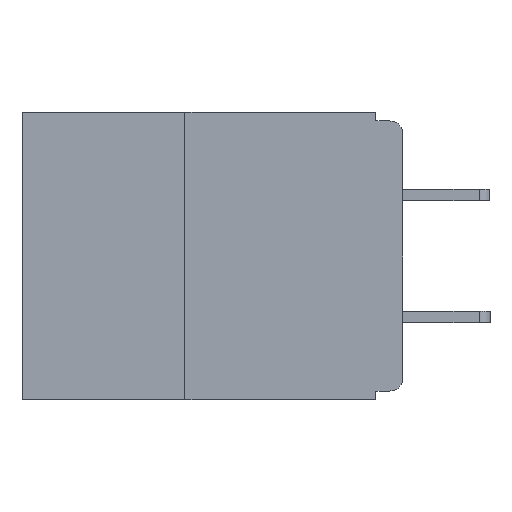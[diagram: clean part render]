
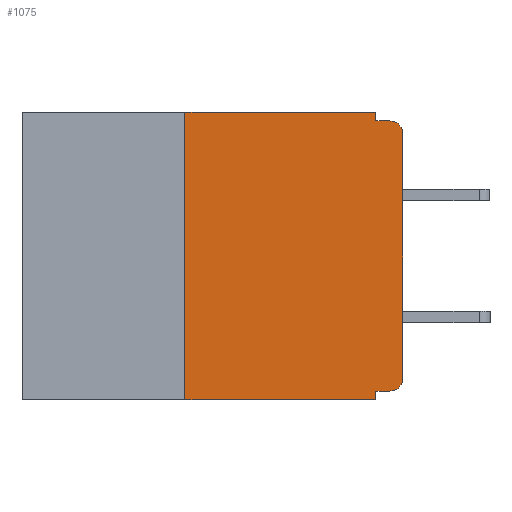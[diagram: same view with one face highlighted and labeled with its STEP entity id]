
A CAD part, left-side view. The second image highlights one B-rep face of the part: STEP entity #1075.
In plain terms, the highlighted planar face has unit normal (-1, 0, 0).
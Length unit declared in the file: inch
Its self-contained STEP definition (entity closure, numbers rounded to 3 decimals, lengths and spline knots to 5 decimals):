
#1011 = EDGE_CURVE ( 'NONE', #8571, #1750, #12185, .T. ) ;
#1016 = AXIS2_PLACEMENT_3D ( 'NONE', #9507, #27413, #12088 ) ;
#1075 = ADVANCED_FACE ( 'NONE', ( #30123 ), #23916, .F. ) ;
#1129 = CARTESIAN_POINT ( 'NONE',  ( 0., 0., -0.32 ) ) ;
#1750 = VERTEX_POINT ( 'NONE', #6474 ) ;
#1765 = DIRECTION ( 'NONE',  ( 0., -1., 0. ) ) ;
#2654 = VECTOR ( 'NONE', #26760, 39.37008 ) ;
#2728 = EDGE_CURVE ( 'NONE', #8571, #25056, #12857, .T. ) ;
#2996 = CIRCLE ( 'NONE', #1016, 0.015 ) ;
#3087 = VERTEX_POINT ( 'NONE', #29708 ) ;
#3171 = AXIS2_PLACEMENT_3D ( 'NONE', #19712, #4345, #22251 ) ;
#3306 = VECTOR ( 'NONE', #9178, 39.37008 ) ;
#3473 = DIRECTION ( 'NONE',  ( 0., -1., 0. ) ) ;
#3576 = CARTESIAN_POINT ( 'NONE',  ( 0., 0., -0.025 ) ) ;
#4042 = DIRECTION ( 'NONE',  ( 0., 0., -1. ) ) ;
#4345 = DIRECTION ( 'NONE',  ( -1., 0., 0. ) ) ;
#5026 = VERTEX_POINT ( 'NONE', #8257 ) ;
#6057 = VECTOR ( 'NONE', #32510, 39.37008 ) ;
#6474 = CARTESIAN_POINT ( 'NONE',  ( 0., 0.031, -0.33 ) ) ;
#6475 = LINE ( 'NONE', #31098, #26116 ) ;
#8257 = CARTESIAN_POINT ( 'NONE',  ( 0., 0.031, -0.32 ) ) ;
#8416 = CARTESIAN_POINT ( 'NONE',  ( 0., 0.25, 0. ) ) ;
#8571 = VERTEX_POINT ( 'NONE', #17820 ) ;
#8887 = EDGE_CURVE ( 'NONE', #3087, #15823, #16781, .T. ) ;
#9062 = CARTESIAN_POINT ( 'NONE',  ( 0., 0.031, 0. ) ) ;
#9178 = DIRECTION ( 'NONE',  ( 0., 0., -1. ) ) ;
#9458 = LINE ( 'NONE', #1129, #2654 ) ;
#9496 = DIRECTION ( 'NONE',  ( 1., 0., 0. ) ) ;
#9507 = CARTESIAN_POINT ( 'NONE',  ( 0., 0.015, -0.025 ) ) ;
#9511 = EDGE_CURVE ( 'NONE', #25465, #5026, #9458, .T. ) ;
#10718 = CARTESIAN_POINT ( 'NONE',  ( 0., 0.25, -0.33 ) ) ;
#10850 = DIRECTION ( 'NONE',  ( 0., 0., -1. ) ) ;
#11037 = ORIENTED_EDGE ( 'NONE', *, *, #9511, .F. ) ;
#11296 = EDGE_CURVE ( 'NONE', #22761, #3087, #31227, .T. ) ;
#11572 = AXIS2_PLACEMENT_3D ( 'NONE', #27772, #9496, #10850 ) ;
#11676 = EDGE_CURVE ( 'NONE', #12655, #16746, #6475, .T. ) ;
#11770 = CIRCLE ( 'NONE', #3171, 0.015 ) ;
#12088 = DIRECTION ( 'NONE',  ( 0., 0., -1. ) ) ;
#12185 = LINE ( 'NONE', #32900, #25022 ) ;
#12477 = VECTOR ( 'NONE', #4042, 39.37008 ) ;
#12655 = VERTEX_POINT ( 'NONE', #20913 ) ;
#12857 = LINE ( 'NONE', #10718, #6057 ) ;
#14676 = ORIENTED_EDGE ( 'NONE', *, *, #21113, .F. ) ;
#15087 = CARTESIAN_POINT ( 'NONE',  ( 0., 0.015, -0.01 ) ) ;
#15823 = VERTEX_POINT ( 'NONE', #15087 ) ;
#16555 = CARTESIAN_POINT ( 'NONE',  ( 0., 0., -0.01 ) ) ;
#16746 = VERTEX_POINT ( 'NONE', #3576 ) ;
#16781 = LINE ( 'NONE', #16555, #22734 ) ;
#17820 = CARTESIAN_POINT ( 'NONE',  ( 0., 0.25, -0.33 ) ) ;
#17947 = VECTOR ( 'NONE', #1765, 39.37008 ) ;
#18492 = DIRECTION ( 'NONE',  ( 0., 0., 1. ) ) ;
#18744 = LINE ( 'NONE', #27363, #17947 ) ;
#19380 = CARTESIAN_POINT ( 'NONE',  ( 0., 0.031, 0. ) ) ;
#19712 = CARTESIAN_POINT ( 'NONE',  ( 0., 0.015, -0.305 ) ) ;
#20913 = CARTESIAN_POINT ( 'NONE',  ( 0., 0., -0.305 ) ) ;
#21113 = EDGE_CURVE ( 'NONE', #25056, #22761, #18744, .T. ) ;
#21466 = ORIENTED_EDGE ( 'NONE', *, *, #2728, .F. ) ;
#21568 = EDGE_LOOP ( 'NONE', ( #22652, #30168, #24259, #31716, #14676, #21466, #22277, #29793, #11037, #31350 ) ) ;
#22180 = EDGE_CURVE ( 'NONE', #16746, #15823, #2996, .T. ) ;
#22251 = DIRECTION ( 'NONE',  ( 0., 0., -1. ) ) ;
#22277 = ORIENTED_EDGE ( 'NONE', *, *, #1011, .T. ) ;
#22652 = ORIENTED_EDGE ( 'NONE', *, *, #11676, .T. ) ;
#22734 = VECTOR ( 'NONE', #31691, 39.37008 ) ;
#22761 = VERTEX_POINT ( 'NONE', #19380 ) ;
#22814 = EDGE_CURVE ( 'NONE', #25465, #12655, #11770, .T. ) ;
#23916 = PLANE ( 'NONE',  #11572 ) ;
#24259 = ORIENTED_EDGE ( 'NONE', *, *, #8887, .F. ) ;
#25022 = VECTOR ( 'NONE', #3473, 39.37008 ) ;
#25056 = VERTEX_POINT ( 'NONE', #8416 ) ;
#25306 = LINE ( 'NONE', #29587, #12477 ) ;
#25389 = CARTESIAN_POINT ( 'NONE',  ( 0., 0.015, -0.32 ) ) ;
#25465 = VERTEX_POINT ( 'NONE', #25389 ) ;
#26116 = VECTOR ( 'NONE', #18492, 39.37008 ) ;
#26760 = DIRECTION ( 'NONE',  ( 0., 1., 0. ) ) ;
#27363 = CARTESIAN_POINT ( 'NONE',  ( 0., 0.437, 0. ) ) ;
#27413 = DIRECTION ( 'NONE',  ( -1., 0., 0. ) ) ;
#27772 = CARTESIAN_POINT ( 'NONE',  ( 0., 0.437, 0. ) ) ;
#29059 = EDGE_CURVE ( 'NONE', #5026, #1750, #25306, .T. ) ;
#29587 = CARTESIAN_POINT ( 'NONE',  ( 0., 0.031, -0.33 ) ) ;
#29708 = CARTESIAN_POINT ( 'NONE',  ( 0., 0.031, -0.01 ) ) ;
#29793 = ORIENTED_EDGE ( 'NONE', *, *, #29059, .F. ) ;
#30123 = FACE_OUTER_BOUND ( 'NONE', #21568, .T. ) ;
#30168 = ORIENTED_EDGE ( 'NONE', *, *, #22180, .T. ) ;
#31098 = CARTESIAN_POINT ( 'NONE',  ( 0., 0., 0. ) ) ;
#31227 = LINE ( 'NONE', #9062, #3306 ) ;
#31350 = ORIENTED_EDGE ( 'NONE', *, *, #22814, .T. ) ;
#31691 = DIRECTION ( 'NONE',  ( 0., -1., 0. ) ) ;
#31716 = ORIENTED_EDGE ( 'NONE', *, *, #11296, .F. ) ;
#32510 = DIRECTION ( 'NONE',  ( 0., 0., 1. ) ) ;
#32900 = CARTESIAN_POINT ( 'NONE',  ( 0., 0.437, -0.33 ) ) ;
